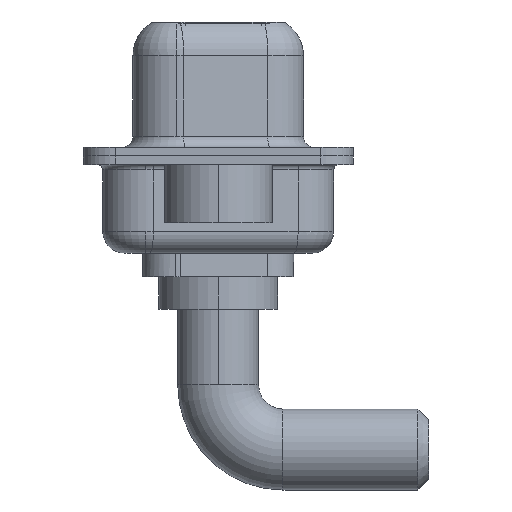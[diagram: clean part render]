
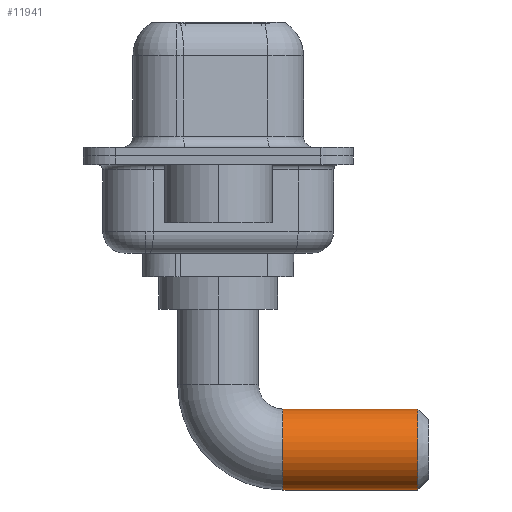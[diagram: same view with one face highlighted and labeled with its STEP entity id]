
A CAD part, left-side view. The second image highlights one B-rep face of the part: STEP entity #11941.
In plain terms, the highlighted cylindrical face has radius 1.875 mm (diameter 3.75 mm), a partial arc.
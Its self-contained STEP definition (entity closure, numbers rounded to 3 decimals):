
#103 = FACE_OUTER_BOUND ( 'NONE', #7061, .T. ) ;
#536 = CIRCLE ( 'NONE', #6894, 1.875 ) ;
#911 = AXIS2_PLACEMENT_3D ( 'NONE', #10130, #10002, #8073 ) ;
#1102 = EDGE_CURVE ( 'NONE', #5015, #7544, #1728, .T. ) ;
#1279 = DIRECTION ( 'NONE',  ( -1., 0., 0. ) ) ;
#1346 = CARTESIAN_POINT ( 'NONE',  ( 0., -3., -4.625 ) ) ;
#1358 = ORIENTED_EDGE ( 'NONE', *, *, #6956, .F. ) ;
#1728 = LINE ( 'NONE', #8270, #2994 ) ;
#2227 = DIRECTION ( 'NONE',  ( 0., 0., -1. ) ) ;
#2755 = ORIENTED_EDGE ( 'NONE', *, *, #5931, .T. ) ;
#2994 = VECTOR ( 'NONE', #7257, 1000. ) ;
#3540 = LINE ( 'NONE', #5767, #5295 ) ;
#3549 = AXIS2_PLACEMENT_3D ( 'NONE', #8813, #9810, #2227 ) ;
#3637 = ORIENTED_EDGE ( 'NONE', *, *, #7618, .T. ) ;
#4132 = DIRECTION ( 'NONE',  ( 0., -1., 0. ) ) ;
#5015 = VERTEX_POINT ( 'NONE', #11096 ) ;
#5295 = VECTOR ( 'NONE', #7573, 1000. ) ;
#5767 = CARTESIAN_POINT ( 'NONE',  ( 0., -3., -4.625 ) ) ;
#5931 = EDGE_CURVE ( 'NONE', #7544, #12136, #6658, .T. ) ;
#5948 = CARTESIAN_POINT ( 'NONE',  ( 0., -3., -6.5 ) ) ;
#6658 = CIRCLE ( 'NONE', #911, 1.875 ) ;
#6894 = AXIS2_PLACEMENT_3D ( 'NONE', #5948, #4132, #1279 ) ;
#6956 = EDGE_CURVE ( 'NONE', #12116, #12136, #3540, .T. ) ;
#7061 = EDGE_LOOP ( 'NONE', ( #1358, #3637, #8357, #2755 ) ) ;
#7257 = DIRECTION ( 'NONE',  ( 0., -1., 0. ) ) ;
#7544 = VERTEX_POINT ( 'NONE', #9364 ) ;
#7573 = DIRECTION ( 'NONE',  ( 0., -1., 0. ) ) ;
#7618 = EDGE_CURVE ( 'NONE', #12116, #5015, #536, .T. ) ;
#8009 = CARTESIAN_POINT ( 'NONE',  ( 0., -9.25, -4.625 ) ) ;
#8073 = DIRECTION ( 'NONE',  ( 0., 0., -1. ) ) ;
#8270 = CARTESIAN_POINT ( 'NONE',  ( 0., -3., -8.375 ) ) ;
#8357 = ORIENTED_EDGE ( 'NONE', *, *, #1102, .T. ) ;
#8813 = CARTESIAN_POINT ( 'NONE',  ( 0., -3., -6.5 ) ) ;
#9364 = CARTESIAN_POINT ( 'NONE',  ( 0., -9.25, -8.375 ) ) ;
#9690 = CYLINDRICAL_SURFACE ( 'NONE', #3549, 1.875 ) ;
#9810 = DIRECTION ( 'NONE',  ( 0., -1., 0. ) ) ;
#10002 = DIRECTION ( 'NONE',  ( 0., 1., 0. ) ) ;
#10130 = CARTESIAN_POINT ( 'NONE',  ( 0., -9.25, -6.5 ) ) ;
#11096 = CARTESIAN_POINT ( 'NONE',  ( 0., -3., -8.375 ) ) ;
#11941 = ADVANCED_FACE ( 'NONE', ( #103 ), #9690, .T. ) ;
#12116 = VERTEX_POINT ( 'NONE', #1346 ) ;
#12136 = VERTEX_POINT ( 'NONE', #8009 ) ;
